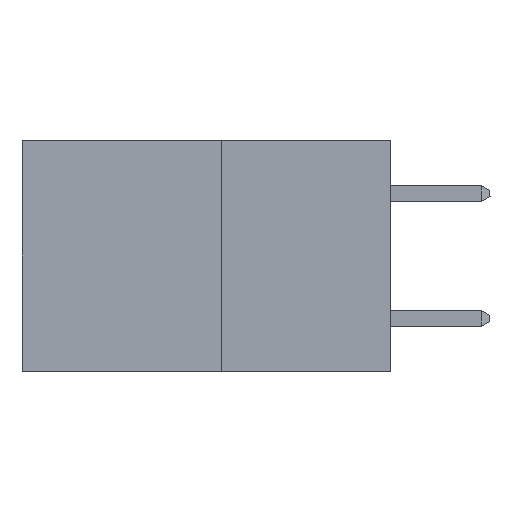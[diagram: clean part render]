
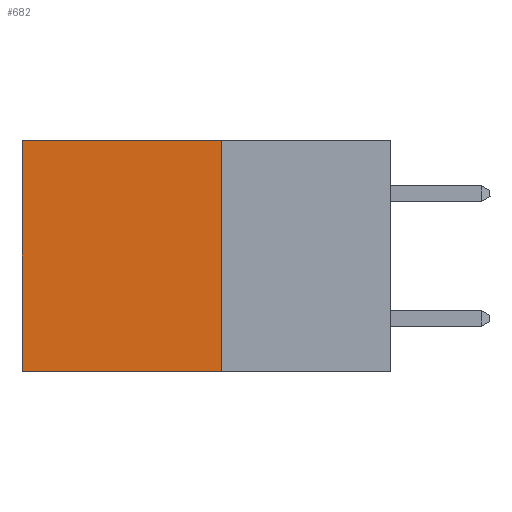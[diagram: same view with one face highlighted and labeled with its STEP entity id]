
A CAD part, left-side view. The second image highlights one B-rep face of the part: STEP entity #682.
In plain terms, the highlighted planar face has unit normal (-1, 0, 0).
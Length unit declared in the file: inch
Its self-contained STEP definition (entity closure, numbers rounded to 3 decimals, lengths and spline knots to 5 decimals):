
#287 = CARTESIAN_POINT ( 'NONE',  ( 0.277, 0.27, -0.37 ) ) ;
#467 = VERTEX_POINT ( 'NONE', #824 ) ;
#478 = VECTOR ( 'NONE', #2570, 39.37008 ) ;
#682 = ADVANCED_FACE ( 'NONE', ( #14851 ), #6876, .F. ) ;
#724 = ORIENTED_EDGE ( 'NONE', *, *, #10662, .F. ) ;
#746 = CARTESIAN_POINT ( 'NONE',  ( 0.277, 0.27, 0. ) ) ;
#824 = CARTESIAN_POINT ( 'NONE',  ( 0.277, 0.59, 0. ) ) ;
#1098 = CARTESIAN_POINT ( 'NONE',  ( 0.277, 0.27, -0.37 ) ) ;
#1488 = ORIENTED_EDGE ( 'NONE', *, *, #5814, .T. ) ;
#2570 = DIRECTION ( 'NONE',  ( 0., 0., -1. ) ) ;
#5011 = EDGE_CURVE ( 'NONE', #9242, #467, #14607, .T. ) ;
#5412 = CARTESIAN_POINT ( 'NONE',  ( 0.277, 0.27, -0.37 ) ) ;
#5814 = EDGE_CURVE ( 'NONE', #467, #13054, #5966, .T. ) ;
#5966 = LINE ( 'NONE', #17849, #8382 ) ;
#6876 = PLANE ( 'NONE',  #13201 ) ;
#6972 = CARTESIAN_POINT ( 'NONE',  ( 0.277, 0.59, -0.37 ) ) ;
#8201 = DIRECTION ( 'NONE',  ( 0., 0., -1. ) ) ;
#8312 = LINE ( 'NONE', #1098, #478 ) ;
#8382 = VECTOR ( 'NONE', #8201, 39.37008 ) ;
#8711 = EDGE_CURVE ( 'NONE', #9242, #16887, #8312, .T. ) ;
#9162 = EDGE_LOOP ( 'NONE', ( #1488, #724, #13275, #12332 ) ) ;
#9242 = VERTEX_POINT ( 'NONE', #746 ) ;
#9319 = CARTESIAN_POINT ( 'NONE',  ( 0.277, 0.27, 0. ) ) ;
#10389 = CARTESIAN_POINT ( 'NONE',  ( 0.277, 0.27, -0.37 ) ) ;
#10624 = DIRECTION ( 'NONE',  ( 1., 0., 0. ) ) ;
#10662 = EDGE_CURVE ( 'NONE', #16887, #13054, #18140, .T. ) ;
#10846 = VECTOR ( 'NONE', #12145, 39.37008 ) ;
#12145 = DIRECTION ( 'NONE',  ( 0., 1., 0. ) ) ;
#12332 = ORIENTED_EDGE ( 'NONE', *, *, #5011, .T. ) ;
#13054 = VERTEX_POINT ( 'NONE', #6972 ) ;
#13201 = AXIS2_PLACEMENT_3D ( 'NONE', #5412, #10624, #15083 ) ;
#13275 = ORIENTED_EDGE ( 'NONE', *, *, #8711, .F. ) ;
#14607 = LINE ( 'NONE', #9319, #10846 ) ;
#14667 = VECTOR ( 'NONE', #16174, 39.37008 ) ;
#14851 = FACE_OUTER_BOUND ( 'NONE', #9162, .T. ) ;
#15083 = DIRECTION ( 'NONE',  ( 0., 0., -1. ) ) ;
#16174 = DIRECTION ( 'NONE',  ( 0., 1., 0. ) ) ;
#16887 = VERTEX_POINT ( 'NONE', #10389 ) ;
#17849 = CARTESIAN_POINT ( 'NONE',  ( 0.277, 0.59, -0.37 ) ) ;
#18140 = LINE ( 'NONE', #287, #14667 ) ;
